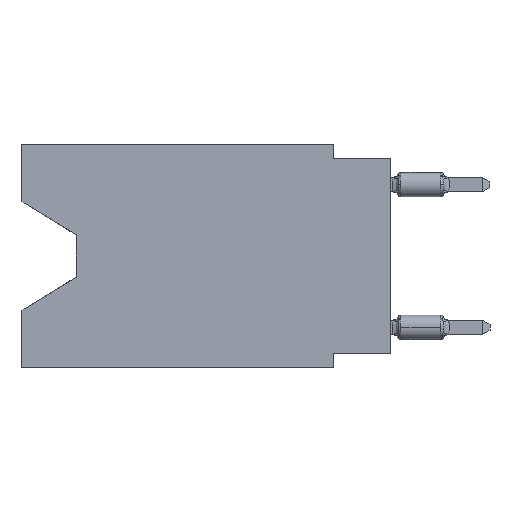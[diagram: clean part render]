
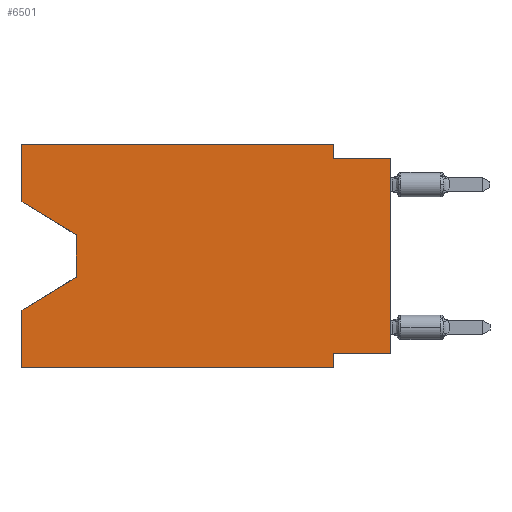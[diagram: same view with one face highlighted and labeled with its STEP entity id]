
A CAD part, left-side view. The second image highlights one B-rep face of the part: STEP entity #6501.
In plain terms, the highlighted planar face has unit normal (-1, 0, 0).
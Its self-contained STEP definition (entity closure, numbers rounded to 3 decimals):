
#98 = CARTESIAN_POINT ( 'NONE',  ( 0., 16.383, -2.546 ) ) ;
#280 = ORIENTED_EDGE ( 'NONE', *, *, #2597, .T. ) ;
#568 = ORIENTED_EDGE ( 'NONE', *, *, #3177, .F. ) ;
#635 = VECTOR ( 'NONE', #931, 1000. ) ;
#666 = EDGE_CURVE ( 'NONE', #6021, #1042, #5779, .T. ) ;
#797 = VECTOR ( 'NONE', #6215, 1000. ) ;
#931 = DIRECTION ( 'NONE',  ( 0., 1., 0. ) ) ;
#948 = VERTEX_POINT ( 'NONE', #12405 ) ;
#959 = VECTOR ( 'NONE', #8215, 1000. ) ;
#963 = CARTESIAN_POINT ( 'NONE',  ( 0., 2.54, -9.906 ) ) ;
#1042 = VERTEX_POINT ( 'NONE', #963 ) ;
#1063 = LINE ( 'NONE', #3956, #635 ) ;
#1175 = VECTOR ( 'NONE', #12244, 1000. ) ;
#1350 = CARTESIAN_POINT ( 'NONE',  ( 0., 2.54, 0. ) ) ;
#1369 = DIRECTION ( 'NONE',  ( 0., 0., 1. ) ) ;
#1522 = ORIENTED_EDGE ( 'NONE', *, *, #2609, .F. ) ;
#1734 = LINE ( 'NONE', #11916, #8147 ) ;
#2113 = VERTEX_POINT ( 'NONE', #3595 ) ;
#2125 = CARTESIAN_POINT ( 'NONE',  ( 0., 16.383, 0. ) ) ;
#2150 = VERTEX_POINT ( 'NONE', #5513 ) ;
#2234 = AXIS2_PLACEMENT_3D ( 'NONE', #5618, #7897, #4036 ) ;
#2342 = LINE ( 'NONE', #11267, #797 ) ;
#2597 = EDGE_CURVE ( 'NONE', #5885, #4818, #6350, .T. ) ;
#2609 = EDGE_CURVE ( 'NONE', #2113, #4818, #7700, .T. ) ;
#2722 = VERTEX_POINT ( 'NONE', #4697 ) ;
#2805 = CARTESIAN_POINT ( 'NONE',  ( 0., 2.54, -9.271 ) ) ;
#2871 = ORIENTED_EDGE ( 'NONE', *, *, #5846, .T. ) ;
#3038 = EDGE_CURVE ( 'NONE', #9783, #5169, #3699, .T. ) ;
#3059 = VECTOR ( 'NONE', #6950, 1000. ) ;
#3139 = CARTESIAN_POINT ( 'NONE',  ( 0., 16.383, -7.36 ) ) ;
#3177 = EDGE_CURVE ( 'NONE', #2722, #2150, #5081, .T. ) ;
#3248 = EDGE_CURVE ( 'NONE', #5885, #6021, #1063, .T. ) ;
#3317 = DIRECTION ( 'NONE',  ( 0., -1., 0. ) ) ;
#3376 = VERTEX_POINT ( 'NONE', #8533 ) ;
#3595 = CARTESIAN_POINT ( 'NONE',  ( 0., 2.54, -0.635 ) ) ;
#3699 = LINE ( 'NONE', #11836, #5214 ) ;
#3771 = CARTESIAN_POINT ( 'NONE',  ( 0., 0., -0.635 ) ) ;
#3946 = ORIENTED_EDGE ( 'NONE', *, *, #666, .F. ) ;
#3956 = CARTESIAN_POINT ( 'NONE',  ( 0., 0., -9.271 ) ) ;
#4036 = DIRECTION ( 'NONE',  ( 0., 0., -1. ) ) ;
#4171 = LINE ( 'NONE', #8099, #4319 ) ;
#4319 = VECTOR ( 'NONE', #3317, 1000. ) ;
#4697 = CARTESIAN_POINT ( 'NONE',  ( 0., 16.383, -2.546 ) ) ;
#4818 = VERTEX_POINT ( 'NONE', #7648 ) ;
#5081 = LINE ( 'NONE', #2125, #959 ) ;
#5169 = VERTEX_POINT ( 'NONE', #3139 ) ;
#5214 = VECTOR ( 'NONE', #12689, 1000. ) ;
#5498 = VERTEX_POINT ( 'NONE', #7294 ) ;
#5513 = CARTESIAN_POINT ( 'NONE',  ( 0., 16.383, 0. ) ) ;
#5618 = CARTESIAN_POINT ( 'NONE',  ( 0., 16.383, 0. ) ) ;
#5779 = LINE ( 'NONE', #7925, #3059 ) ;
#5784 = VECTOR ( 'NONE', #6203, 1000. ) ;
#5806 = ORIENTED_EDGE ( 'NONE', *, *, #3248, .F. ) ;
#5846 = EDGE_CURVE ( 'NONE', #948, #3376, #8386, .T. ) ;
#5885 = VERTEX_POINT ( 'NONE', #7472 ) ;
#5943 = EDGE_LOOP ( 'NONE', ( #9616, #2871, #10027, #6436, #7134, #3946, #5806, #280, #1522, #6230, #7372, #568 ) ) ;
#6021 = VERTEX_POINT ( 'NONE', #2805 ) ;
#6203 = DIRECTION ( 'NONE',  ( 0., 0., -1. ) ) ;
#6215 = DIRECTION ( 'NONE',  ( 0., 0.855, -0.519 ) ) ;
#6230 = ORIENTED_EDGE ( 'NONE', *, *, #6638, .F. ) ;
#6350 = LINE ( 'NONE', #12397, #7995 ) ;
#6436 = ORIENTED_EDGE ( 'NONE', *, *, #3038, .F. ) ;
#6501 = ADVANCED_FACE ( 'NONE', ( #11476 ), #10601, .F. ) ;
#6556 = CARTESIAN_POINT ( 'NONE',  ( 0., 16.383, -9.906 ) ) ;
#6638 = EDGE_CURVE ( 'NONE', #5498, #2113, #9208, .T. ) ;
#6665 = EDGE_CURVE ( 'NONE', #2722, #948, #10407, .T. ) ;
#6681 = EDGE_CURVE ( 'NONE', #9783, #1042, #4171, .T. ) ;
#6849 = VECTOR ( 'NONE', #7280, 1000. ) ;
#6950 = DIRECTION ( 'NONE',  ( 0., 0., -1. ) ) ;
#7134 = ORIENTED_EDGE ( 'NONE', *, *, #6681, .T. ) ;
#7280 = DIRECTION ( 'NONE',  ( 0., 0., -1. ) ) ;
#7294 = CARTESIAN_POINT ( 'NONE',  ( 0., 2.54, 0. ) ) ;
#7372 = ORIENTED_EDGE ( 'NONE', *, *, #7447, .F. ) ;
#7447 = EDGE_CURVE ( 'NONE', #2150, #5498, #1734, .T. ) ;
#7472 = CARTESIAN_POINT ( 'NONE',  ( 0., 0., -9.271 ) ) ;
#7648 = CARTESIAN_POINT ( 'NONE',  ( 0., 0., -0.635 ) ) ;
#7700 = LINE ( 'NONE', #3771, #10318 ) ;
#7897 = DIRECTION ( 'NONE',  ( 1., 0., 0. ) ) ;
#7925 = CARTESIAN_POINT ( 'NONE',  ( 0., 2.54, -9.906 ) ) ;
#7995 = VECTOR ( 'NONE', #1369, 1000. ) ;
#8099 = CARTESIAN_POINT ( 'NONE',  ( 0., 16.383, -9.906 ) ) ;
#8147 = VECTOR ( 'NONE', #10790, 1000. ) ;
#8215 = DIRECTION ( 'NONE',  ( 0., 0., 1. ) ) ;
#8386 = LINE ( 'NONE', #11356, #6849 ) ;
#8533 = CARTESIAN_POINT ( 'NONE',  ( 0., 13.97, -5.893 ) ) ;
#8837 = EDGE_CURVE ( 'NONE', #3376, #5169, #2342, .T. ) ;
#9208 = LINE ( 'NONE', #1350, #5784 ) ;
#9616 = ORIENTED_EDGE ( 'NONE', *, *, #6665, .T. ) ;
#9783 = VERTEX_POINT ( 'NONE', #6556 ) ;
#9806 = DIRECTION ( 'NONE',  ( 0., -1., 0. ) ) ;
#10027 = ORIENTED_EDGE ( 'NONE', *, *, #8837, .T. ) ;
#10318 = VECTOR ( 'NONE', #9806, 1000. ) ;
#10407 = LINE ( 'NONE', #98, #1175 ) ;
#10601 = PLANE ( 'NONE',  #2234 ) ;
#10790 = DIRECTION ( 'NONE',  ( 0., -1., 0. ) ) ;
#11267 = CARTESIAN_POINT ( 'NONE',  ( 0., 13.97, -5.893 ) ) ;
#11356 = CARTESIAN_POINT ( 'NONE',  ( 0., 13.97, -4.013 ) ) ;
#11476 = FACE_OUTER_BOUND ( 'NONE', #5943, .T. ) ;
#11836 = CARTESIAN_POINT ( 'NONE',  ( 0., 16.383, 0. ) ) ;
#11916 = CARTESIAN_POINT ( 'NONE',  ( 0., 16.383, 0. ) ) ;
#12244 = DIRECTION ( 'NONE',  ( 0., -0.855, -0.519 ) ) ;
#12397 = CARTESIAN_POINT ( 'NONE',  ( 0., 0., 0. ) ) ;
#12405 = CARTESIAN_POINT ( 'NONE',  ( 0., 13.97, -4.013 ) ) ;
#12689 = DIRECTION ( 'NONE',  ( 0., 0., 1. ) ) ;
